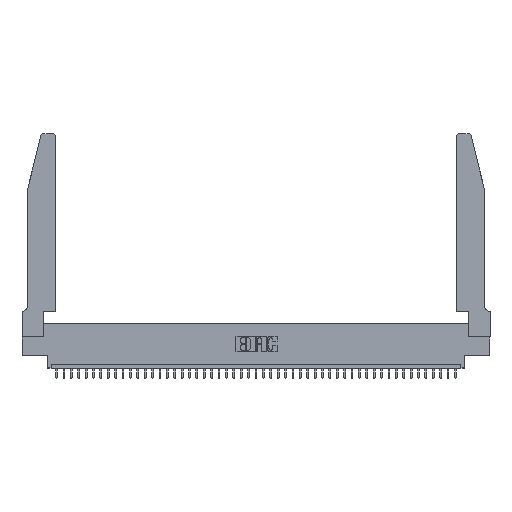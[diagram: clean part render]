
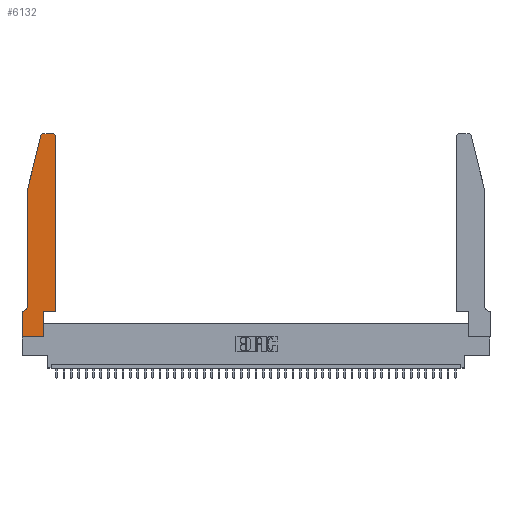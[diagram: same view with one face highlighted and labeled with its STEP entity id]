
A CAD part, top view. The second image highlights one B-rep face of the part: STEP entity #6132.
In plain terms, the highlighted planar face has unit normal (0, 0, 1).
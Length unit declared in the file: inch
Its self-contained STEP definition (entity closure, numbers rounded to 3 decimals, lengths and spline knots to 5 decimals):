
#1098 = VECTOR ( 'NONE', #39122, 39.37008 ) ;
#1336 = VECTOR ( 'NONE', #8406, 39.37008 ) ;
#2173 = DIRECTION ( 'NONE',  ( 1., 0., 0. ) ) ;
#2398 = CARTESIAN_POINT ( 'NONE',  ( 0.4505, 0.35, 0.37 ) ) ;
#2674 = ORIENTED_EDGE ( 'NONE', *, *, #15993, .T. ) ;
#2691 = VECTOR ( 'NONE', #12060, 39.37008 ) ;
#3593 = DIRECTION ( 'NONE',  ( 0., -1., 0. ) ) ;
#4868 = VERTEX_POINT ( 'NONE', #43017 ) ;
#5195 = EDGE_CURVE ( 'NONE', #44556, #28421, #19813, .T. ) ;
#6111 = CARTESIAN_POINT ( 'NONE',  ( 0.0755, 0.35, 0.37 ) ) ;
#6132 = ADVANCED_FACE ( 'NONE', ( #19167 ), #36068, .T. ) ;
#6242 = CARTESIAN_POINT ( 'NONE',  ( 0.0755, 2., 0.37 ) ) ;
#6949 = LINE ( 'NONE', #31567, #41407 ) ;
#7586 = ORIENTED_EDGE ( 'NONE', *, *, #40815, .T. ) ;
#8406 = DIRECTION ( 'NONE',  ( -1., 0., 0. ) ) ;
#8793 = DIRECTION ( 'NONE',  ( 1., 0., 0. ) ) ;
#8846 = LINE ( 'NONE', #9272, #19091 ) ;
#9029 = CARTESIAN_POINT ( 'NONE',  ( 0.4205, 2.72, 0.37 ) ) ;
#9175 = VERTEX_POINT ( 'NONE', #38902 ) ;
#9213 = VERTEX_POINT ( 'NONE', #27214 ) ;
#9272 = CARTESIAN_POINT ( 'NONE',  ( 0., 0., 0.37 ) ) ;
#11163 = VECTOR ( 'NONE', #43338, 39.37008 ) ;
#12060 = DIRECTION ( 'NONE',  ( 0., 1., 0. ) ) ;
#12875 = CIRCLE ( 'NONE', #41825, 0.07 ) ;
#13642 = CARTESIAN_POINT ( 'NONE',  ( 0.0755, 0.42, 0.37 ) ) ;
#14047 = ORIENTED_EDGE ( 'NONE', *, *, #29623, .T. ) ;
#14747 = CIRCLE ( 'NONE', #26745, 0.03 ) ;
#15628 = DIRECTION ( 'NONE',  ( -1., 0., 0. ) ) ;
#15993 = EDGE_CURVE ( 'NONE', #18230, #35214, #32484, .T. ) ;
#16475 = DIRECTION ( 'NONE',  ( 0., 0., 1. ) ) ;
#16487 = ORIENTED_EDGE ( 'NONE', *, *, #25222, .T. ) ;
#17972 = EDGE_LOOP ( 'NONE', ( #16487, #14047, #35938, #27458, #38332, #38874, #19175, #26733, #7586, #2674, #41340, #31148 ) ) ;
#18230 = VERTEX_POINT ( 'NONE', #22983 ) ;
#18386 = LINE ( 'NONE', #32804, #2691 ) ;
#18528 = VERTEX_POINT ( 'NONE', #19497 ) ;
#19091 = VECTOR ( 'NONE', #2173, 39.37008 ) ;
#19167 = FACE_OUTER_BOUND ( 'NONE', #17972, .T. ) ;
#19175 = ORIENTED_EDGE ( 'NONE', *, *, #29160, .T. ) ;
#19497 = CARTESIAN_POINT ( 'NONE',  ( 0.25487, 2.72718, 0.37 ) ) ;
#19813 = LINE ( 'NONE', #6242, #36535 ) ;
#21918 = DIRECTION ( 'NONE',  ( 0., 1., 0. ) ) ;
#22769 = EDGE_CURVE ( 'NONE', #28421, #26749, #12875, .T. ) ;
#22983 = CARTESIAN_POINT ( 'NONE',  ( 0.2865, 0.35, 0.37 ) ) ;
#24091 = EDGE_CURVE ( 'NONE', #18528, #44556, #26224, .T. ) ;
#25137 = CARTESIAN_POINT ( 'NONE',  ( 0., 0., 0.37 ) ) ;
#25222 = EDGE_CURVE ( 'NONE', #42870, #36350, #26649, .T. ) ;
#25893 = AXIS2_PLACEMENT_3D ( 'NONE', #32446, #36221, #8793 ) ;
#26224 = LINE ( 'NONE', #39763, #11163 ) ;
#26372 = DIRECTION ( 'NONE',  ( 1., 0., 0. ) ) ;
#26572 = CARTESIAN_POINT ( 'NONE',  ( 0.2865, 0., 0.37 ) ) ;
#26621 = DIRECTION ( 'NONE',  ( 1., 0., 0. ) ) ;
#26649 = LINE ( 'NONE', #29041, #1336 ) ;
#26733 = ORIENTED_EDGE ( 'NONE', *, *, #38926, .T. ) ;
#26745 = AXIS2_PLACEMENT_3D ( 'NONE', #9029, #33248, #26621 ) ;
#26749 = VERTEX_POINT ( 'NONE', #42602 ) ;
#27214 = CARTESIAN_POINT ( 'NONE',  ( 0.4505, 2.72, 0.37 ) ) ;
#27458 = ORIENTED_EDGE ( 'NONE', *, *, #5195, .T. ) ;
#27511 = LINE ( 'NONE', #25137, #1098 ) ;
#28326 = VERTEX_POINT ( 'NONE', #26572 ) ;
#28421 = VERTEX_POINT ( 'NONE', #13642 ) ;
#29041 = CARTESIAN_POINT ( 'NONE',  ( 0.2605, 2.75, 0.37 ) ) ;
#29160 = EDGE_CURVE ( 'NONE', #9175, #4868, #27511, .T. ) ;
#29619 = CIRCLE ( 'NONE', #38422, 0.03 ) ;
#29623 = EDGE_CURVE ( 'NONE', #36350, #18528, #29619, .T. ) ;
#30315 = CARTESIAN_POINT ( 'NONE',  ( 0.284, 2.72, 0.37 ) ) ;
#31148 = ORIENTED_EDGE ( 'NONE', *, *, #35262, .T. ) ;
#31461 = CARTESIAN_POINT ( 'NONE',  ( 0.0755, 2., 0.37 ) ) ;
#31495 = EDGE_CURVE ( 'NONE', #26749, #9175, #40682, .T. ) ;
#31567 = CARTESIAN_POINT ( 'NONE',  ( 0.4505, 0.35, 0.37 ) ) ;
#32446 = CARTESIAN_POINT ( 'NONE',  ( 0., 0.35, 0.37 ) ) ;
#32484 = LINE ( 'NONE', #2398, #41104 ) ;
#32804 = CARTESIAN_POINT ( 'NONE',  ( 0.2865, 0.35, 0.37 ) ) ;
#33248 = DIRECTION ( 'NONE',  ( 0., 0., 1. ) ) ;
#33396 = CARTESIAN_POINT ( 'NONE',  ( 0.4505, 0.35, 0.37 ) ) ;
#34816 = VECTOR ( 'NONE', #36828, 39.37008 ) ;
#35214 = VERTEX_POINT ( 'NONE', #33396 ) ;
#35262 = EDGE_CURVE ( 'NONE', #9213, #42870, #14747, .T. ) ;
#35938 = ORIENTED_EDGE ( 'NONE', *, *, #24091, .T. ) ;
#36068 = PLANE ( 'NONE',  #25893 ) ;
#36221 = DIRECTION ( 'NONE',  ( 0., 0., 1. ) ) ;
#36263 = DIRECTION ( 'NONE',  ( 0., 0., -1. ) ) ;
#36350 = VERTEX_POINT ( 'NONE', #42731 ) ;
#36535 = VECTOR ( 'NONE', #3593, 39.37008 ) ;
#36828 = DIRECTION ( 'NONE',  ( -1., 0., 0. ) ) ;
#38332 = ORIENTED_EDGE ( 'NONE', *, *, #22769, .T. ) ;
#38422 = AXIS2_PLACEMENT_3D ( 'NONE', #30315, #16475, #44208 ) ;
#38874 = ORIENTED_EDGE ( 'NONE', *, *, #31495, .T. ) ;
#38902 = CARTESIAN_POINT ( 'NONE',  ( 0., 0.35, 0.37 ) ) ;
#38926 = EDGE_CURVE ( 'NONE', #4868, #28326, #8846, .T. ) ;
#39122 = DIRECTION ( 'NONE',  ( 0., -1., 0. ) ) ;
#39520 = CARTESIAN_POINT ( 'NONE',  ( 0.0055, 0.42, 0.37 ) ) ;
#39763 = CARTESIAN_POINT ( 'NONE',  ( 0.0755, 2., 0.37 ) ) ;
#40682 = LINE ( 'NONE', #6111, #34816 ) ;
#40815 = EDGE_CURVE ( 'NONE', #28326, #18230, #18386, .T. ) ;
#41104 = VECTOR ( 'NONE', #26372, 39.37008 ) ;
#41229 = CARTESIAN_POINT ( 'NONE',  ( 0.4205, 2.75, 0.37 ) ) ;
#41340 = ORIENTED_EDGE ( 'NONE', *, *, #41875, .T. ) ;
#41407 = VECTOR ( 'NONE', #21918, 39.37008 ) ;
#41825 = AXIS2_PLACEMENT_3D ( 'NONE', #39520, #36263, #15628 ) ;
#41875 = EDGE_CURVE ( 'NONE', #35214, #9213, #6949, .T. ) ;
#42602 = CARTESIAN_POINT ( 'NONE',  ( 0.0055, 0.35, 0.37 ) ) ;
#42731 = CARTESIAN_POINT ( 'NONE',  ( 0.284, 2.75, 0.37 ) ) ;
#42870 = VERTEX_POINT ( 'NONE', #41229 ) ;
#43017 = CARTESIAN_POINT ( 'NONE',  ( 0., 0., 0.37 ) ) ;
#43338 = DIRECTION ( 'NONE',  ( -0.239, -0.971, 0. ) ) ;
#44208 = DIRECTION ( 'NONE',  ( 1., 0., 0. ) ) ;
#44556 = VERTEX_POINT ( 'NONE', #31461 ) ;
